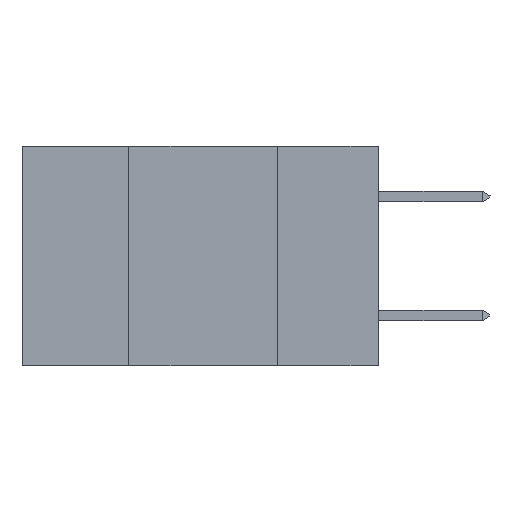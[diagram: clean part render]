
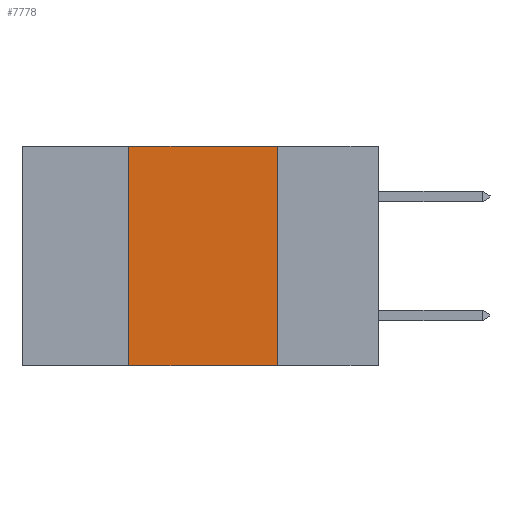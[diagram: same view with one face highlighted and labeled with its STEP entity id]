
A CAD part, left-side view. The second image highlights one B-rep face of the part: STEP entity #7778.
In plain terms, the highlighted planar face has unit normal (-1, 0, 0).
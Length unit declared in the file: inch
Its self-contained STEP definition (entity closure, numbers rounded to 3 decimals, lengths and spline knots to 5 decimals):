
#950 = DIRECTION ( 'NONE',  ( 0., 0., 1. ) ) ;
#1214 = PLANE ( 'NONE',  #12326 ) ;
#1672 = DIRECTION ( 'NONE',  ( 0., 0., -1. ) ) ;
#1901 = CARTESIAN_POINT ( 'NONE',  ( 0., 0.17, -0.37 ) ) ;
#2092 = CARTESIAN_POINT ( 'NONE',  ( 0., 0.6, -0.37 ) ) ;
#2701 = FACE_OUTER_BOUND ( 'NONE', #10330, .T. ) ;
#3719 = CARTESIAN_POINT ( 'NONE',  ( 0., 0.42, -0.37 ) ) ;
#4538 = VERTEX_POINT ( 'NONE', #13859 ) ;
#4711 = CARTESIAN_POINT ( 'NONE',  ( 0., 0.6, 0. ) ) ;
#5996 = VERTEX_POINT ( 'NONE', #16639 ) ;
#6231 = CARTESIAN_POINT ( 'NONE',  ( 0., 0.17, -0.37 ) ) ;
#6688 = VECTOR ( 'NONE', #1672, 39.37008 ) ;
#6805 = LINE ( 'NONE', #3719, #11356 ) ;
#7263 = CARTESIAN_POINT ( 'NONE',  ( 0., 0.6, 0. ) ) ;
#7778 = ADVANCED_FACE ( 'NONE', ( #2701 ), #1214, .F. ) ;
#7822 = VERTEX_POINT ( 'NONE', #1901 ) ;
#8497 = VERTEX_POINT ( 'NONE', #16216 ) ;
#8599 = EDGE_CURVE ( 'NONE', #8497, #4538, #14428, .T. ) ;
#8838 = DIRECTION ( 'NONE',  ( 0., 0., -1. ) ) ;
#10128 = EDGE_CURVE ( 'NONE', #4538, #7822, #15429, .T. ) ;
#10330 = EDGE_LOOP ( 'NONE', ( #13710, #18035, #13887, #19419 ) ) ;
#11228 = EDGE_CURVE ( 'NONE', #5996, #8497, #6805, .T. ) ;
#11356 = VECTOR ( 'NONE', #950, 39.37008 ) ;
#12326 = AXIS2_PLACEMENT_3D ( 'NONE', #7263, #13306, #8838 ) ;
#13306 = DIRECTION ( 'NONE',  ( 1., 0., 0. ) ) ;
#13710 = ORIENTED_EDGE ( 'NONE', *, *, #10128, .F. ) ;
#13859 = CARTESIAN_POINT ( 'NONE',  ( 0., 0.17, 0. ) ) ;
#13887 = ORIENTED_EDGE ( 'NONE', *, *, #11228, .F. ) ;
#14428 = LINE ( 'NONE', #4711, #16453 ) ;
#15429 = LINE ( 'NONE', #6231, #6688 ) ;
#15748 = EDGE_CURVE ( 'NONE', #5996, #7822, #18847, .T. ) ;
#16216 = CARTESIAN_POINT ( 'NONE',  ( 0., 0.42, 0. ) ) ;
#16453 = VECTOR ( 'NONE', #18190, 39.37008 ) ;
#16639 = CARTESIAN_POINT ( 'NONE',  ( 0., 0.42, -0.37 ) ) ;
#16680 = VECTOR ( 'NONE', #16975, 39.37008 ) ;
#16975 = DIRECTION ( 'NONE',  ( 0., -1., 0. ) ) ;
#18035 = ORIENTED_EDGE ( 'NONE', *, *, #8599, .F. ) ;
#18190 = DIRECTION ( 'NONE',  ( 0., -1., 0. ) ) ;
#18847 = LINE ( 'NONE', #2092, #16680 ) ;
#19419 = ORIENTED_EDGE ( 'NONE', *, *, #15748, .T. ) ;
